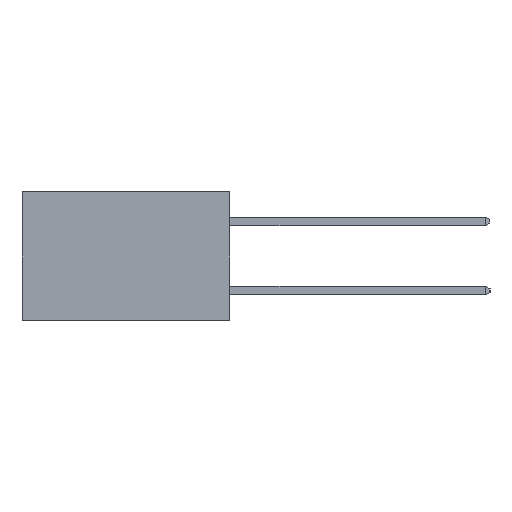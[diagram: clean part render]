
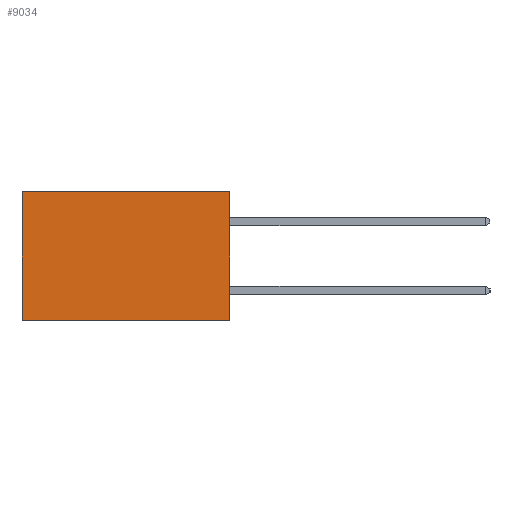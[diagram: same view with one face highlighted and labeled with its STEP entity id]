
A CAD part, left-side view. The second image highlights one B-rep face of the part: STEP entity #9034.
In plain terms, the highlighted planar face has unit normal (-1, 0, 0).
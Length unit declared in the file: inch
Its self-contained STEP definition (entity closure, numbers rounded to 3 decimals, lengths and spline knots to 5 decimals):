
#98 = CARTESIAN_POINT ( 'NONE',  ( 0.2615, 0., 0. ) ) ;
#659 = CARTESIAN_POINT ( 'NONE',  ( 0.2615, 0., -0.37 ) ) ;
#1247 = CARTESIAN_POINT ( 'NONE',  ( 0.2615, 0., -0.37 ) ) ;
#1420 = CARTESIAN_POINT ( 'NONE',  ( 0.2615, 0., -0.37 ) ) ;
#1997 = DIRECTION ( 'NONE',  ( 0., 0., -1. ) ) ;
#2147 = VERTEX_POINT ( 'NONE', #98 ) ;
#2947 = VERTEX_POINT ( 'NONE', #5001 ) ;
#3495 = LINE ( 'NONE', #5023, #6904 ) ;
#3585 = CARTESIAN_POINT ( 'NONE',  ( 0.2615, 0.6, 0. ) ) ;
#4693 = VECTOR ( 'NONE', #7973, 39.37008 ) ;
#5001 = CARTESIAN_POINT ( 'NONE',  ( 0.2615, 0.6, -0.37 ) ) ;
#5023 = CARTESIAN_POINT ( 'NONE',  ( 0.2615, 0., -0.37 ) ) ;
#5448 = VERTEX_POINT ( 'NONE', #1247 ) ;
#5853 = VECTOR ( 'NONE', #11416, 39.37008 ) ;
#6351 = ORIENTED_EDGE ( 'NONE', *, *, #15180, .F. ) ;
#6904 = VECTOR ( 'NONE', #13618, 39.37008 ) ;
#7173 = PLANE ( 'NONE',  #7766 ) ;
#7548 = EDGE_CURVE ( 'NONE', #2147, #15817, #11300, .T. ) ;
#7689 = CARTESIAN_POINT ( 'NONE',  ( 0.2615, 0., 0. ) ) ;
#7766 = AXIS2_PLACEMENT_3D ( 'NONE', #659, #9639, #1997 ) ;
#7973 = DIRECTION ( 'NONE',  ( 0., 1., 0. ) ) ;
#9034 = ADVANCED_FACE ( 'NONE', ( #12025 ), #7173, .F. ) ;
#9102 = DIRECTION ( 'NONE',  ( 0., 0., -1. ) ) ;
#9143 = LINE ( 'NONE', #10181, #5853 ) ;
#9615 = ORIENTED_EDGE ( 'NONE', *, *, #7548, .T. ) ;
#9639 = DIRECTION ( 'NONE',  ( 1., 0., 0. ) ) ;
#10181 = CARTESIAN_POINT ( 'NONE',  ( 0.2615, 0.6, -0.37 ) ) ;
#10628 = EDGE_CURVE ( 'NONE', #15817, #2947, #9143, .T. ) ;
#10714 = EDGE_CURVE ( 'NONE', #2147, #5448, #14081, .T. ) ;
#11263 = VECTOR ( 'NONE', #9102, 39.37008 ) ;
#11300 = LINE ( 'NONE', #7689, #4693 ) ;
#11416 = DIRECTION ( 'NONE',  ( 0., 0., -1. ) ) ;
#12025 = FACE_OUTER_BOUND ( 'NONE', #14957, .T. ) ;
#12422 = ORIENTED_EDGE ( 'NONE', *, *, #10628, .T. ) ;
#13618 = DIRECTION ( 'NONE',  ( 0., 1., 0. ) ) ;
#13767 = ORIENTED_EDGE ( 'NONE', *, *, #10714, .F. ) ;
#14081 = LINE ( 'NONE', #1420, #11263 ) ;
#14957 = EDGE_LOOP ( 'NONE', ( #12422, #6351, #13767, #9615 ) ) ;
#15180 = EDGE_CURVE ( 'NONE', #5448, #2947, #3495, .T. ) ;
#15817 = VERTEX_POINT ( 'NONE', #3585 ) ;
